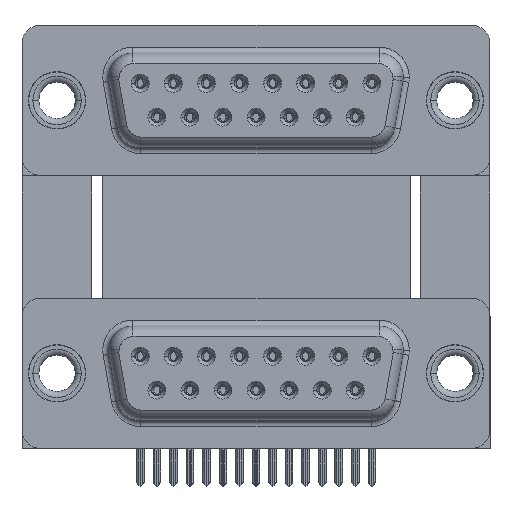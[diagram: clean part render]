
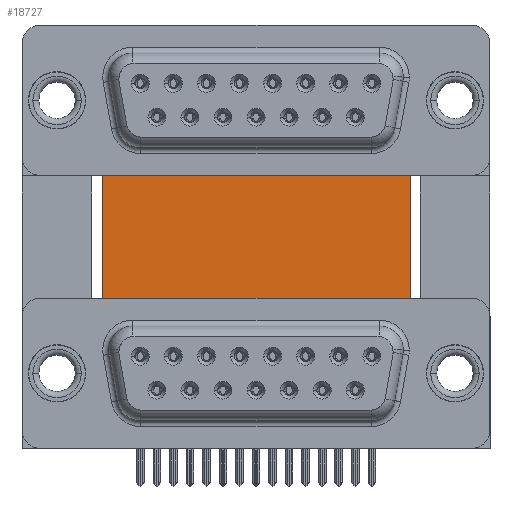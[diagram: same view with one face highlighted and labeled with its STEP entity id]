
A CAD part, top view. The second image highlights one B-rep face of the part: STEP entity #18727.
In plain terms, the highlighted planar face has unit normal (0, 0, 1).
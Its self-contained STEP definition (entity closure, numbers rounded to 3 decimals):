
#763 = DIRECTION ( 'NONE',  ( 0., 0., -1. ) ) ;
#864 = VECTOR ( 'NONE', #14280, 1000. ) ;
#3035 = VECTOR ( 'NONE', #34211, 1000. ) ;
#3750 = LINE ( 'NONE', #18568, #20673 ) ;
#4725 = FACE_OUTER_BOUND ( 'NONE', #4924, .T. ) ;
#4924 = EDGE_LOOP ( 'NONE', ( #17865, #39922, #46684, #9251 ) ) ;
#4969 = AXIS2_PLACEMENT_3D ( 'NONE', #11382, #763, #12112 ) ;
#9251 = ORIENTED_EDGE ( 'NONE', *, *, #18543, .T. ) ;
#10892 = CARTESIAN_POINT ( 'NONE',  ( 29.58, 16.585, -12. ) ) ;
#11382 = CARTESIAN_POINT ( 'NONE',  ( 3.79, 16.585, -12. ) ) ;
#12112 = DIRECTION ( 'NONE',  ( -1., 0., 0. ) ) ;
#13785 = VECTOR ( 'NONE', #23413, 1000. ) ;
#14280 = DIRECTION ( 'NONE',  ( 1., 0., 0. ) ) ;
#15494 = VERTEX_POINT ( 'NONE', #30687 ) ;
#16615 = EDGE_CURVE ( 'NONE', #31123, #39996, #21946, .T. ) ;
#17865 = ORIENTED_EDGE ( 'NONE', *, *, #34981, .T. ) ;
#18543 = EDGE_CURVE ( 'NONE', #31123, #37294, #3750, .T. ) ;
#18568 = CARTESIAN_POINT ( 'NONE',  ( 3.79, 16.585, -12. ) ) ;
#18727 = ADVANCED_FACE ( 'NONE', ( #4725 ), #19777, .F. ) ;
#19777 = PLANE ( 'NONE',  #4969 ) ;
#19955 = CARTESIAN_POINT ( 'NONE',  ( 29.58, 16.585, -12. ) ) ;
#20673 = VECTOR ( 'NONE', #33871, 1000. ) ;
#21946 = LINE ( 'NONE', #37260, #864 ) ;
#23338 = LINE ( 'NONE', #46304, #3035 ) ;
#23413 = DIRECTION ( 'NONE',  ( 0., -1., 0. ) ) ;
#28565 = EDGE_CURVE ( 'NONE', #39996, #15494, #31781, .T. ) ;
#30687 = CARTESIAN_POINT ( 'NONE',  ( 29.58, -3.735, -12. ) ) ;
#31123 = VERTEX_POINT ( 'NONE', #35419 ) ;
#31781 = LINE ( 'NONE', #19955, #13785 ) ;
#33871 = DIRECTION ( 'NONE',  ( 0., -1., 0. ) ) ;
#34211 = DIRECTION ( 'NONE',  ( 1., 0., 0. ) ) ;
#34981 = EDGE_CURVE ( 'NONE', #37294, #15494, #23338, .T. ) ;
#35419 = CARTESIAN_POINT ( 'NONE',  ( 3.79, 16.585, -12. ) ) ;
#36471 = CARTESIAN_POINT ( 'NONE',  ( 3.79, -3.735, -12. ) ) ;
#37260 = CARTESIAN_POINT ( 'NONE',  ( 3.79, 16.585, -12. ) ) ;
#37294 = VERTEX_POINT ( 'NONE', #36471 ) ;
#39922 = ORIENTED_EDGE ( 'NONE', *, *, #28565, .F. ) ;
#39996 = VERTEX_POINT ( 'NONE', #10892 ) ;
#46304 = CARTESIAN_POINT ( 'NONE',  ( 3.79, -3.735, -12. ) ) ;
#46684 = ORIENTED_EDGE ( 'NONE', *, *, #16615, .F. ) ;
